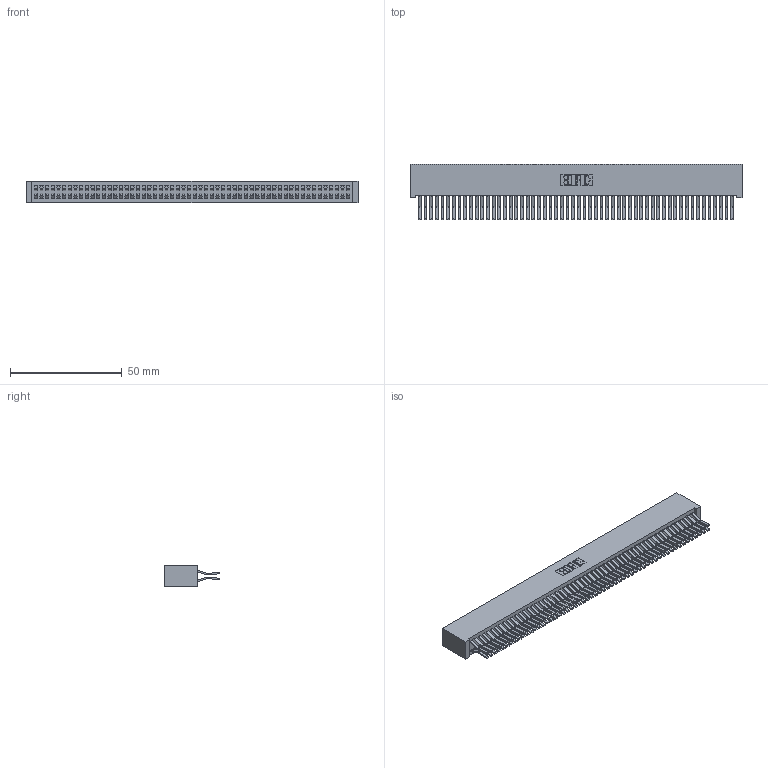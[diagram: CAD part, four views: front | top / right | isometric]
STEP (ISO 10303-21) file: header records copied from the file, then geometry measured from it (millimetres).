
FILE_DESCRIPTION (( 'STEP AP203' ), '1' );
FILE_NAME ('342-112-560-201.STEP', '2018-08-14T12:33:38', ( '' ), ( '' ), 'SwSTEP 2.0', 'SolidWorks 2016', '' );
FILE_SCHEMA (( 'CONFIG_CONTROL_DESIGN' ));
Length unit declared in the file: inch
Products named in the file (3): 342 Part_Lugless; 345-292-001_560 Tail; 342-112-560-201
Assembly tree (113 placements, depth 2):
  342-112-560-201
    342 Part_Lugless
    345-292-001_560 Tail  x112
Bounding box: 148.49 x 24.78 x 9.4 mm (x, y, z)
Volume: 14582.8 mm3; surface area: 26291.5 mm2
Topology: 113 solids, 113 shells, 6150 faces, 18307 edges, 12054 vertices
Faces by surface type: plane 4094, cylinder 2056
Entity records: 33895 total; most frequent: CARTESIAN_POINT 5598, ORIENTED_EDGE 5534, DIRECTION 4755, EDGE_CURVE 2767, LINE 2643, VECTOR 2643, VERTEX_POINT 1842, AXIS2_PLACEMENT_3D 1056
